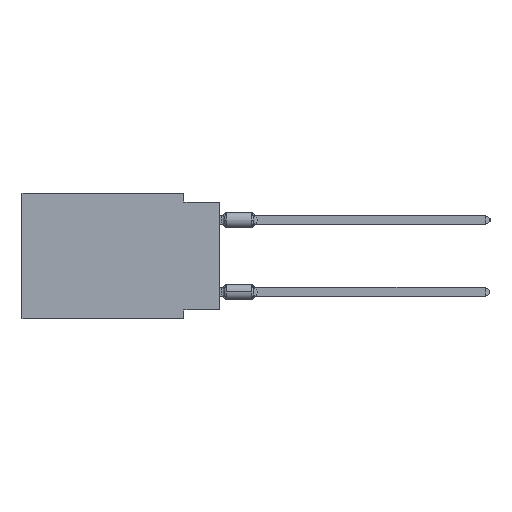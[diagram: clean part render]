
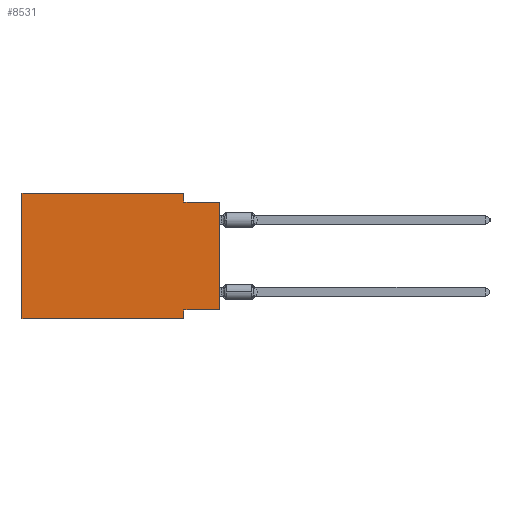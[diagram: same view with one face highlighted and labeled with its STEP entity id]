
A CAD part, left-side view. The second image highlights one B-rep face of the part: STEP entity #8531.
In plain terms, the highlighted planar face has unit normal (-1, 0, 0).
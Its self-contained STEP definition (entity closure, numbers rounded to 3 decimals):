
#533 = CARTESIAN_POINT ( 'NONE',  ( 0., 13.97, -8.89 ) ) ;
#1221 = VECTOR ( 'NONE', #24073, 1000. ) ;
#1306 = CARTESIAN_POINT ( 'NONE',  ( 0., 2.54, -0.635 ) ) ;
#2210 = ORIENTED_EDGE ( 'NONE', *, *, #9884, .F. ) ;
#3386 = VERTEX_POINT ( 'NONE', #8584 ) ;
#4569 = DIRECTION ( 'NONE',  ( 0., 0., -1. ) ) ;
#4574 = LINE ( 'NONE', #6587, #14075 ) ;
#4640 = VERTEX_POINT ( 'NONE', #8166 ) ;
#5824 = VERTEX_POINT ( 'NONE', #1306 ) ;
#6060 = LINE ( 'NONE', #29335, #17674 ) ;
#6587 = CARTESIAN_POINT ( 'NONE',  ( 0., 0., -0.635 ) ) ;
#6885 = DIRECTION ( 'NONE',  ( 1., 0., 0. ) ) ;
#7930 = LINE ( 'NONE', #15479, #9781 ) ;
#7983 = VERTEX_POINT ( 'NONE', #29450 ) ;
#8166 = CARTESIAN_POINT ( 'NONE',  ( 0., 2.54, -8.89 ) ) ;
#8531 = ADVANCED_FACE ( 'NONE', ( #9202 ), #18620, .F. ) ;
#8584 = CARTESIAN_POINT ( 'NONE',  ( 0., 13.97, -8.89 ) ) ;
#9008 = EDGE_CURVE ( 'NONE', #7983, #4640, #15126, .T. ) ;
#9142 = VECTOR ( 'NONE', #9653, 1000. ) ;
#9202 = FACE_OUTER_BOUND ( 'NONE', #17505, .T. ) ;
#9653 = DIRECTION ( 'NONE',  ( 0., 1., 0. ) ) ;
#9670 = EDGE_CURVE ( 'NONE', #5824, #18265, #4574, .T. ) ;
#9723 = ORIENTED_EDGE ( 'NONE', *, *, #15986, .F. ) ;
#9781 = VECTOR ( 'NONE', #17331, 1000. ) ;
#9884 = EDGE_CURVE ( 'NONE', #29858, #7983, #12420, .T. ) ;
#10787 = ORIENTED_EDGE ( 'NONE', *, *, #14974, .F. ) ;
#11560 = AXIS2_PLACEMENT_3D ( 'NONE', #27998, #6885, #4569 ) ;
#12420 = LINE ( 'NONE', #21839, #9142 ) ;
#12563 = LINE ( 'NONE', #533, #24772 ) ;
#12993 = CARTESIAN_POINT ( 'NONE',  ( 0., 13.97, 0. ) ) ;
#13684 = CARTESIAN_POINT ( 'NONE',  ( 0., 2.54, 0. ) ) ;
#13740 = VERTEX_POINT ( 'NONE', #12993 ) ;
#13754 = ORIENTED_EDGE ( 'NONE', *, *, #17769, .T. ) ;
#14075 = VECTOR ( 'NONE', #18625, 1000. ) ;
#14505 = CARTESIAN_POINT ( 'NONE',  ( 0., 2.54, -8.89 ) ) ;
#14566 = DIRECTION ( 'NONE',  ( 0., -1., 0. ) ) ;
#14734 = ORIENTED_EDGE ( 'NONE', *, *, #9670, .F. ) ;
#14907 = VECTOR ( 'NONE', #21517, 1000. ) ;
#14974 = EDGE_CURVE ( 'NONE', #13740, #16460, #6060, .T. ) ;
#15126 = LINE ( 'NONE', #14505, #1221 ) ;
#15479 = CARTESIAN_POINT ( 'NONE',  ( 0., 13.97, 0. ) ) ;
#15986 = EDGE_CURVE ( 'NONE', #16460, #5824, #25389, .T. ) ;
#16279 = CARTESIAN_POINT ( 'NONE',  ( 0., 0., 0. ) ) ;
#16460 = VERTEX_POINT ( 'NONE', #16969 ) ;
#16540 = CARTESIAN_POINT ( 'NONE',  ( 0., 0., -8.255 ) ) ;
#16969 = CARTESIAN_POINT ( 'NONE',  ( 0., 2.54, 0. ) ) ;
#17331 = DIRECTION ( 'NONE',  ( 0., 0., 1. ) ) ;
#17505 = EDGE_LOOP ( 'NONE', ( #13754, #14734, #9723, #10787, #22253, #29684, #18096, #2210 ) ) ;
#17674 = VECTOR ( 'NONE', #29939, 1000. ) ;
#17769 = EDGE_CURVE ( 'NONE', #29858, #18265, #28135, .T. ) ;
#17846 = EDGE_CURVE ( 'NONE', #3386, #4640, #12563, .T. ) ;
#18096 = ORIENTED_EDGE ( 'NONE', *, *, #9008, .F. ) ;
#18265 = VERTEX_POINT ( 'NONE', #21782 ) ;
#18620 = PLANE ( 'NONE',  #11560 ) ;
#18625 = DIRECTION ( 'NONE',  ( 0., -1., 0. ) ) ;
#21517 = DIRECTION ( 'NONE',  ( 0., 0., 1. ) ) ;
#21782 = CARTESIAN_POINT ( 'NONE',  ( 0., 0., -0.635 ) ) ;
#21839 = CARTESIAN_POINT ( 'NONE',  ( 0., 0., -8.255 ) ) ;
#22253 = ORIENTED_EDGE ( 'NONE', *, *, #25986, .F. ) ;
#23099 = DIRECTION ( 'NONE',  ( 0., 0., -1. ) ) ;
#23220 = VECTOR ( 'NONE', #23099, 1000. ) ;
#24073 = DIRECTION ( 'NONE',  ( 0., 0., -1. ) ) ;
#24772 = VECTOR ( 'NONE', #14566, 1000. ) ;
#25389 = LINE ( 'NONE', #13684, #23220 ) ;
#25986 = EDGE_CURVE ( 'NONE', #3386, #13740, #7930, .T. ) ;
#27998 = CARTESIAN_POINT ( 'NONE',  ( 0., 13.97, 0. ) ) ;
#28135 = LINE ( 'NONE', #16279, #14907 ) ;
#29335 = CARTESIAN_POINT ( 'NONE',  ( 0., 13.97, 0. ) ) ;
#29450 = CARTESIAN_POINT ( 'NONE',  ( 0., 2.54, -8.255 ) ) ;
#29684 = ORIENTED_EDGE ( 'NONE', *, *, #17846, .T. ) ;
#29858 = VERTEX_POINT ( 'NONE', #16540 ) ;
#29939 = DIRECTION ( 'NONE',  ( 0., -1., 0. ) ) ;
